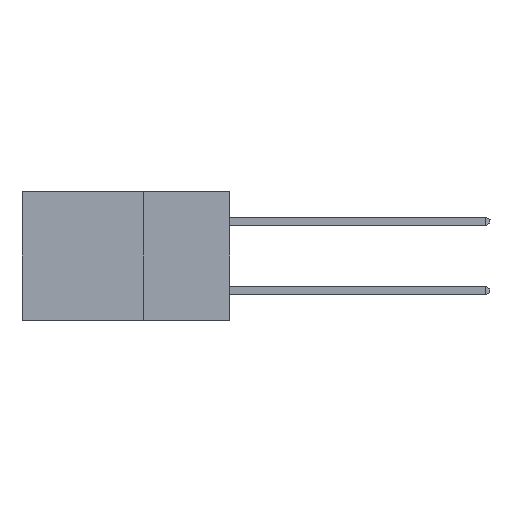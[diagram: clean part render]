
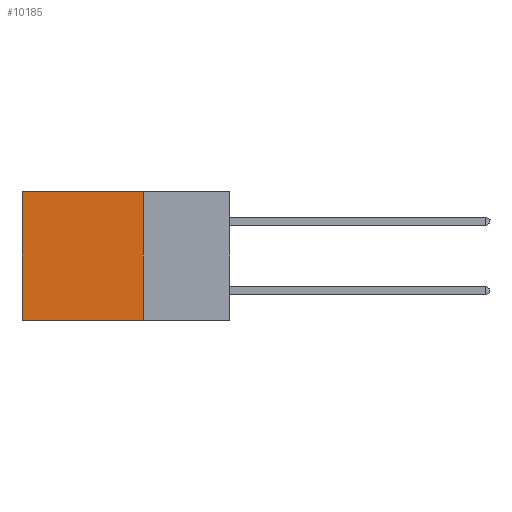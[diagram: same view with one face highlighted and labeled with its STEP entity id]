
A CAD part, left-side view. The second image highlights one B-rep face of the part: STEP entity #10185.
In plain terms, the highlighted planar face has unit normal (-1, 0, 0).
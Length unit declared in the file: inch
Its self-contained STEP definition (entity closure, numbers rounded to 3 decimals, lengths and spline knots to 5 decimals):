
#1201 = VECTOR ( 'NONE', #13569, 39.37008 ) ;
#1824 = VERTEX_POINT ( 'NONE', #15199 ) ;
#2844 = EDGE_LOOP ( 'NONE', ( #3984, #16750, #8863, #11405 ) ) ;
#2867 = VERTEX_POINT ( 'NONE', #21461 ) ;
#3984 = ORIENTED_EDGE ( 'NONE', *, *, #16277, .T. ) ;
#7033 = EDGE_CURVE ( 'NONE', #9412, #18908, #15509, .T. ) ;
#7069 = CARTESIAN_POINT ( 'NONE',  ( 0.298, 0.25, 0. ) ) ;
#7445 = DIRECTION ( 'NONE',  ( 0., 0., -1. ) ) ;
#8471 = LINE ( 'NONE', #9338, #14052 ) ;
#8863 = ORIENTED_EDGE ( 'NONE', *, *, #7033, .F. ) ;
#9263 = CARTESIAN_POINT ( 'NONE',  ( 0.298, 0.25, 0. ) ) ;
#9338 = CARTESIAN_POINT ( 'NONE',  ( 0.298, 0.25, 0. ) ) ;
#9412 = VERTEX_POINT ( 'NONE', #7069 ) ;
#10185 = ADVANCED_FACE ( 'NONE', ( #21472 ), #20611, .F. ) ;
#11405 = ORIENTED_EDGE ( 'NONE', *, *, #20582, .T. ) ;
#11425 = CARTESIAN_POINT ( 'NONE',  ( 0.298, 0.25, -0.37 ) ) ;
#12452 = DIRECTION ( 'NONE',  ( 0., 1., 0. ) ) ;
#13066 = CARTESIAN_POINT ( 'NONE',  ( 0.298, 0.25, 0. ) ) ;
#13569 = DIRECTION ( 'NONE',  ( 0., 1., 0. ) ) ;
#14052 = VECTOR ( 'NONE', #12452, 39.37008 ) ;
#14901 = CARTESIAN_POINT ( 'NONE',  ( 0.298, 0.25, -0.37 ) ) ;
#15199 = CARTESIAN_POINT ( 'NONE',  ( 0.298, 0.6, 0. ) ) ;
#15509 = LINE ( 'NONE', #13066, #19026 ) ;
#16277 = EDGE_CURVE ( 'NONE', #1824, #2867, #21767, .T. ) ;
#16750 = ORIENTED_EDGE ( 'NONE', *, *, #21052, .F. ) ;
#16807 = VECTOR ( 'NONE', #19936, 39.37008 ) ;
#17244 = LINE ( 'NONE', #11425, #1201 ) ;
#18294 = DIRECTION ( 'NONE',  ( 0., 0., -1. ) ) ;
#18908 = VERTEX_POINT ( 'NONE', #14901 ) ;
#19026 = VECTOR ( 'NONE', #18294, 39.37008 ) ;
#19936 = DIRECTION ( 'NONE',  ( 0., 0., -1. ) ) ;
#20582 = EDGE_CURVE ( 'NONE', #9412, #1824, #8471, .T. ) ;
#20611 = PLANE ( 'NONE',  #21788 ) ;
#21052 = EDGE_CURVE ( 'NONE', #18908, #2867, #17244, .T. ) ;
#21461 = CARTESIAN_POINT ( 'NONE',  ( 0.298, 0.6, -0.37 ) ) ;
#21472 = FACE_OUTER_BOUND ( 'NONE', #2844, .T. ) ;
#21714 = CARTESIAN_POINT ( 'NONE',  ( 0.298, 0.6, 0. ) ) ;
#21767 = LINE ( 'NONE', #21714, #16807 ) ;
#21788 = AXIS2_PLACEMENT_3D ( 'NONE', #9263, #22336, #7445 ) ;
#22336 = DIRECTION ( 'NONE',  ( 1., 0., 0. ) ) ;
